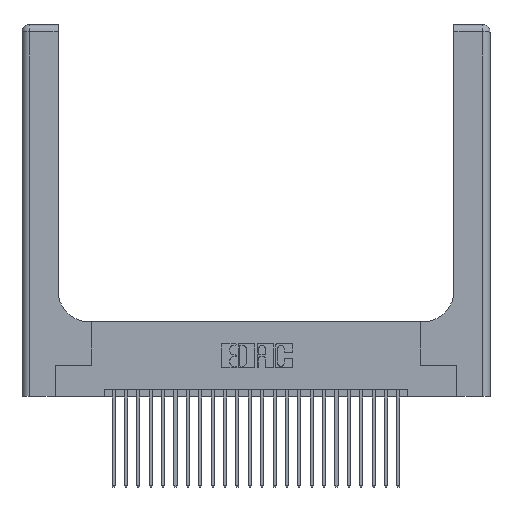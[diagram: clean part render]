
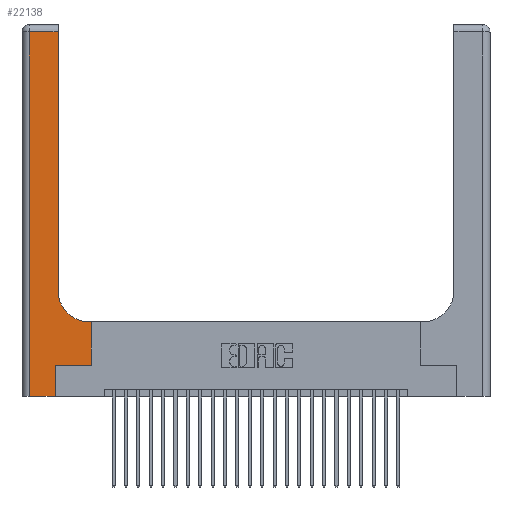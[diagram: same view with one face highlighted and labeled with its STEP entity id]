
A CAD part, top view. The second image highlights one B-rep face of the part: STEP entity #22138.
In plain terms, the highlighted planar face has unit normal (0, 0, 1).
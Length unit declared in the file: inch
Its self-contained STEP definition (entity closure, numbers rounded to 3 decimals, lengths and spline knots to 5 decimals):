
#824 = ORIENTED_EDGE ( 'NONE', *, *, #1878, .T. ) ;
#1415 = EDGE_CURVE ( 'NONE', #23726, #14351, #3574, .T. ) ;
#1501 = LINE ( 'NONE', #25273, #21045 ) ;
#1878 = EDGE_CURVE ( 'NONE', #4726, #15249, #7713, .T. ) ;
#1894 = AXIS2_PLACEMENT_3D ( 'NONE', #10969, #25452, #13235 ) ;
#2052 = VECTOR ( 'NONE', #5134, 39.37008 ) ;
#2153 = ORIENTED_EDGE ( 'NONE', *, *, #10098, .T. ) ;
#2204 = VECTOR ( 'NONE', #10825, 39.37008 ) ;
#2944 = VERTEX_POINT ( 'NONE', #23326 ) ;
#3574 = LINE ( 'NONE', #17182, #16691 ) ;
#3642 = CARTESIAN_POINT ( 'NONE',  ( 0.5585, 0.25, 0.37 ) ) ;
#4664 = ORIENTED_EDGE ( 'NONE', *, *, #20820, .T. ) ;
#4726 = VERTEX_POINT ( 'NONE', #13056 ) ;
#5134 = DIRECTION ( 'NONE',  ( 0., 1., 0. ) ) ;
#5187 = VECTOR ( 'NONE', #26324, 39.37008 ) ;
#6197 = ORIENTED_EDGE ( 'NONE', *, *, #19436, .T. ) ;
#6512 = DIRECTION ( 'NONE',  ( -1., 0., 0. ) ) ;
#6969 = DIRECTION ( 'NONE',  ( 0., 1., 0. ) ) ;
#7056 = LINE ( 'NONE', #14854, #16634 ) ;
#7226 = CARTESIAN_POINT ( 'NONE',  ( 0.2915, 2.94, 0.37 ) ) ;
#7300 = ORIENTED_EDGE ( 'NONE', *, *, #17931, .T. ) ;
#7375 = ORIENTED_EDGE ( 'NONE', *, *, #9768, .T. ) ;
#7568 = LINE ( 'NONE', #15357, #2052 ) ;
#7713 = LINE ( 'NONE', #16942, #2204 ) ;
#7734 = LINE ( 'NONE', #18287, #5187 ) ;
#7925 = VECTOR ( 'NONE', #20240, 39.37008 ) ;
#8060 = CARTESIAN_POINT ( 'NONE',  ( 0.2915, 3., 0.37 ) ) ;
#8744 = ORIENTED_EDGE ( 'NONE', *, *, #1415, .T. ) ;
#9031 = PLANE ( 'NONE',  #1894 ) ;
#9768 = EDGE_CURVE ( 'NONE', #17849, #13915, #26446, .T. ) ;
#10098 = EDGE_CURVE ( 'NONE', #13915, #23726, #23569, .T. ) ;
#10825 = DIRECTION ( 'NONE',  ( 1., 0., 0. ) ) ;
#10969 = CARTESIAN_POINT ( 'NONE',  ( 0., 3., 0.37 ) ) ;
#11084 = CARTESIAN_POINT ( 'NONE',  ( 0.5415, 0.85, 0.37 ) ) ;
#11183 = EDGE_CURVE ( 'NONE', #25129, #17849, #19697, .T. ) ;
#12069 = AXIS2_PLACEMENT_3D ( 'NONE', #11084, #13066, #15048 ) ;
#12693 = DIRECTION ( 'NONE',  ( -1., 0., 0. ) ) ;
#13056 = CARTESIAN_POINT ( 'NONE',  ( 0.269, 0.25, 0.37 ) ) ;
#13066 = DIRECTION ( 'NONE',  ( 0., 0., -1. ) ) ;
#13235 = DIRECTION ( 'NONE',  ( -1., 0., 0. ) ) ;
#13767 = EDGE_CURVE ( 'NONE', #14351, #2944, #7734, .T. ) ;
#13902 = FACE_OUTER_BOUND ( 'NONE', #21712, .T. ) ;
#13915 = VERTEX_POINT ( 'NONE', #7226 ) ;
#13973 = CARTESIAN_POINT ( 'NONE',  ( 0.5585, 0.6, 0.37 ) ) ;
#14351 = VERTEX_POINT ( 'NONE', #20968 ) ;
#14663 = VERTEX_POINT ( 'NONE', #13973 ) ;
#14854 = CARTESIAN_POINT ( 'NONE',  ( 0.2915, 0.6, 0.37 ) ) ;
#14951 = CARTESIAN_POINT ( 'NONE',  ( 0., 2.94, 0.37 ) ) ;
#15048 = DIRECTION ( 'NONE',  ( 1., 0., 0. ) ) ;
#15249 = VERTEX_POINT ( 'NONE', #3642 ) ;
#15357 = CARTESIAN_POINT ( 'NONE',  ( 0.5585, 0.25, 0.37 ) ) ;
#16204 = CARTESIAN_POINT ( 'NONE',  ( 0.06, 2.94, 0.37 ) ) ;
#16225 = VECTOR ( 'NONE', #12693, 39.37008 ) ;
#16634 = VECTOR ( 'NONE', #6512, 39.37008 ) ;
#16691 = VECTOR ( 'NONE', #25453, 39.37008 ) ;
#16942 = CARTESIAN_POINT ( 'NONE',  ( 0.269, 0.25, 0.37 ) ) ;
#17182 = CARTESIAN_POINT ( 'NONE',  ( 0.06, 3., 0.37 ) ) ;
#17849 = VERTEX_POINT ( 'NONE', #25953 ) ;
#17931 = EDGE_CURVE ( 'NONE', #14663, #25129, #7056, .T. ) ;
#18287 = CARTESIAN_POINT ( 'NONE',  ( 0., 0., 0.37 ) ) ;
#19436 = EDGE_CURVE ( 'NONE', #2944, #4726, #1501, .T. ) ;
#19697 = CIRCLE ( 'NONE', #12069, 0.25 ) ;
#20240 = DIRECTION ( 'NONE',  ( 0., 1., 0. ) ) ;
#20415 = ORIENTED_EDGE ( 'NONE', *, *, #13767, .T. ) ;
#20820 = EDGE_CURVE ( 'NONE', #15249, #14663, #7568, .T. ) ;
#20968 = CARTESIAN_POINT ( 'NONE',  ( 0.06, 0., 0.37 ) ) ;
#21045 = VECTOR ( 'NONE', #6969, 39.37008 ) ;
#21712 = EDGE_LOOP ( 'NONE', ( #7375, #2153, #8744, #20415, #6197, #824, #4664, #7300, #26141 ) ) ;
#22138 = ADVANCED_FACE ( 'NONE', ( #13902 ), #9031, .F. ) ;
#22840 = CARTESIAN_POINT ( 'NONE',  ( 0.5415, 0.6, 0.37 ) ) ;
#23326 = CARTESIAN_POINT ( 'NONE',  ( 0.269, 0., 0.37 ) ) ;
#23569 = LINE ( 'NONE', #14951, #16225 ) ;
#23726 = VERTEX_POINT ( 'NONE', #16204 ) ;
#25129 = VERTEX_POINT ( 'NONE', #22840 ) ;
#25273 = CARTESIAN_POINT ( 'NONE',  ( 0.269, 0., 0.37 ) ) ;
#25452 = DIRECTION ( 'NONE',  ( 0., 0., -1. ) ) ;
#25453 = DIRECTION ( 'NONE',  ( 0., -1., 0. ) ) ;
#25953 = CARTESIAN_POINT ( 'NONE',  ( 0.2915, 0.85, 0.37 ) ) ;
#26141 = ORIENTED_EDGE ( 'NONE', *, *, #11183, .T. ) ;
#26324 = DIRECTION ( 'NONE',  ( 1., 0., 0. ) ) ;
#26446 = LINE ( 'NONE', #8060, #7925 ) ;
